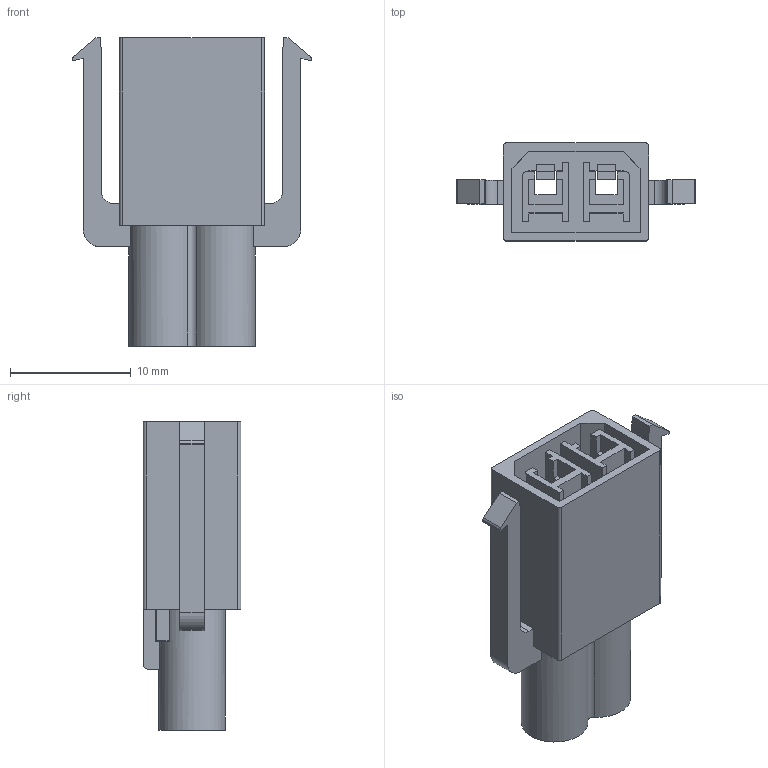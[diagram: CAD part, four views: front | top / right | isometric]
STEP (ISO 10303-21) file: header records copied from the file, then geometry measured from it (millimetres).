
FILE_DESCRIPTION (( 'STEP AP214' ), '1' );
FILE_NAME ('567-002-000-410.STEP', '2020-07-27T19:56:32', ( '' ), ( '' ), 'SwSTEP 2.0', 'SolidWorks 2020', '' );
FILE_SCHEMA (( 'AUTOMOTIVE_DESIGN' ));
Length unit declared in the file: millimetre
Products named in the file (1): 567-002-000-410
Bounding box: 19.8 x 8.1 x 25.5 mm (x, y, z)
Volume: 1010.6 mm3; surface area: 2924.3 mm2
Topology: 1 solids, 1 shells, 196 faces, 565 edges, 372 vertices
Faces by surface type: plane 157, cylinder 31, bspline 6, sphere 2
Entity records: 6731 total; most frequent: CARTESIAN_POINT 1562, ORIENTED_EDGE 1126, DIRECTION 993, EDGE_CURVE 563, LINE 463, VECTOR 463, VERTEX_POINT 372, AXIS2_PLACEMENT_3D 265
